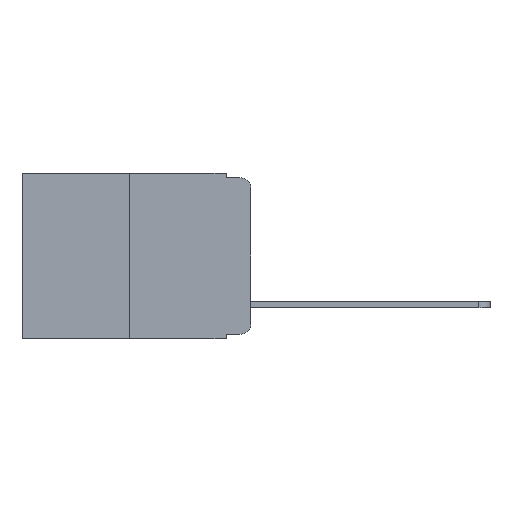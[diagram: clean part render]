
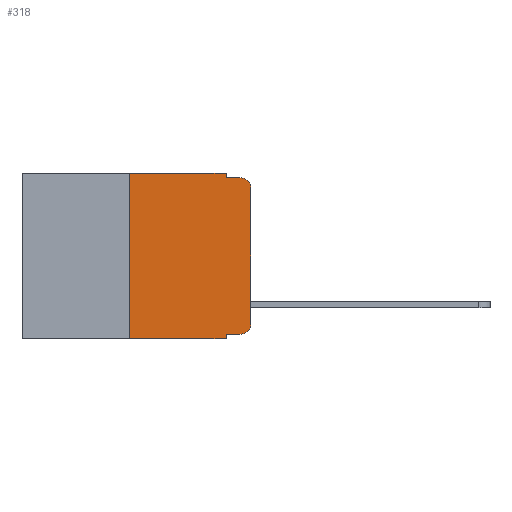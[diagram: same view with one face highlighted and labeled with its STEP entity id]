
A CAD part, left-side view. The second image highlights one B-rep face of the part: STEP entity #318.
In plain terms, the highlighted planar face has unit normal (-1, 0, 0).
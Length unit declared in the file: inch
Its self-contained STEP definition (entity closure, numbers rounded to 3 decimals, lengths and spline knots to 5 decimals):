
#45 = CARTESIAN_POINT ( 'NONE',  ( 0., 0., -0.03 ) ) ;
#90 = DIRECTION ( 'NONE',  ( 0., -1., 0. ) ) ;
#96 = PLANE ( 'NONE',  #7021 ) ;
#160 = ORIENTED_EDGE ( 'NONE', *, *, #5198, .T. ) ;
#318 = ADVANCED_FACE ( 'NONE', ( #749 ), #96, .F. ) ;
#366 = VECTOR ( 'NONE', #1645, 39.37008 ) ;
#488 = VERTEX_POINT ( 'NONE', #9440 ) ;
#749 = FACE_OUTER_BOUND ( 'NONE', #10147, .T. ) ;
#823 = ORIENTED_EDGE ( 'NONE', *, *, #6202, .T. ) ;
#852 = VERTEX_POINT ( 'NONE', #1570 ) ;
#1126 = VERTEX_POINT ( 'NONE', #3689 ) ;
#1153 = LINE ( 'NONE', #7464, #6526 ) ;
#1239 = VERTEX_POINT ( 'NONE', #6737 ) ;
#1570 = CARTESIAN_POINT ( 'NONE',  ( 0., 0.02, -0.01 ) ) ;
#1645 = DIRECTION ( 'NONE',  ( 0., 0., -1. ) ) ;
#1784 = LINE ( 'NONE', #7136, #11660 ) ;
#1896 = CARTESIAN_POINT ( 'NONE',  ( 0., 0., 0. ) ) ;
#2383 = DIRECTION ( 'NONE',  ( 0., 0., 1. ) ) ;
#2514 = CARTESIAN_POINT ( 'NONE',  ( 0., 0.25, 0. ) ) ;
#2850 = VERTEX_POINT ( 'NONE', #11942 ) ;
#3355 = VERTEX_POINT ( 'NONE', #9206 ) ;
#3689 = CARTESIAN_POINT ( 'NONE',  ( 0., 0.051, -0.01 ) ) ;
#3874 = CARTESIAN_POINT ( 'NONE',  ( 0., 0.02, -0.333 ) ) ;
#4204 = VERTEX_POINT ( 'NONE', #45 ) ;
#4306 = DIRECTION ( 'NONE',  ( -1., 0., 0. ) ) ;
#4560 = DIRECTION ( 'NONE',  ( 0., -1., 0. ) ) ;
#4792 = EDGE_CURVE ( 'NONE', #1126, #852, #9647, .T. ) ;
#4904 = CARTESIAN_POINT ( 'NONE',  ( 0., 0.473, -0.343 ) ) ;
#4909 = CARTESIAN_POINT ( 'NONE',  ( 0., 0.051, -0.01 ) ) ;
#5058 = CIRCLE ( 'NONE', #6511, 0.02 ) ;
#5089 = VECTOR ( 'NONE', #8851, 39.37008 ) ;
#5197 = VERTEX_POINT ( 'NONE', #2514 ) ;
#5198 = EDGE_CURVE ( 'NONE', #9395, #4204, #5793, .T. ) ;
#5280 = CIRCLE ( 'NONE', #8051, 0.02 ) ;
#5439 = LINE ( 'NONE', #9256, #12081 ) ;
#5793 = LINE ( 'NONE', #1896, #12102 ) ;
#5828 = VERTEX_POINT ( 'NONE', #3874 ) ;
#6048 = DIRECTION ( 'NONE',  ( 0., -1., 0. ) ) ;
#6202 = EDGE_CURVE ( 'NONE', #4204, #852, #5280, .T. ) ;
#6375 = ORIENTED_EDGE ( 'NONE', *, *, #8945, .T. ) ;
#6511 = AXIS2_PLACEMENT_3D ( 'NONE', #11617, #11629, #6986 ) ;
#6526 = VECTOR ( 'NONE', #8425, 39.37008 ) ;
#6737 = CARTESIAN_POINT ( 'NONE',  ( 0., 0.051, 0. ) ) ;
#6873 = EDGE_CURVE ( 'NONE', #2850, #5197, #5439, .T. ) ;
#6971 = DIRECTION ( 'NONE',  ( 1., 0., 0. ) ) ;
#6986 = DIRECTION ( 'NONE',  ( 0., 0., -1. ) ) ;
#7021 = AXIS2_PLACEMENT_3D ( 'NONE', #7030, #6971, #7131 ) ;
#7030 = CARTESIAN_POINT ( 'NONE',  ( 0., 0.473, 0. ) ) ;
#7092 = ORIENTED_EDGE ( 'NONE', *, *, #8535, .T. ) ;
#7131 = DIRECTION ( 'NONE',  ( 0., 0., -1. ) ) ;
#7136 = CARTESIAN_POINT ( 'NONE',  ( 0., 0.051, -0.333 ) ) ;
#7150 = ORIENTED_EDGE ( 'NONE', *, *, #9022, .F. ) ;
#7186 = ORIENTED_EDGE ( 'NONE', *, *, #11784, .T. ) ;
#7464 = CARTESIAN_POINT ( 'NONE',  ( 0., 0.051, 0. ) ) ;
#8051 = AXIS2_PLACEMENT_3D ( 'NONE', #9296, #4306, #10740 ) ;
#8417 = LINE ( 'NONE', #8868, #366 ) ;
#8425 = DIRECTION ( 'NONE',  ( 0., 0., -1. ) ) ;
#8504 = CARTESIAN_POINT ( 'NONE',  ( 0., 0., -0.313 ) ) ;
#8535 = EDGE_CURVE ( 'NONE', #488, #5828, #1784, .T. ) ;
#8619 = ORIENTED_EDGE ( 'NONE', *, *, #6873, .F. ) ;
#8668 = ORIENTED_EDGE ( 'NONE', *, *, #10211, .F. ) ;
#8851 = DIRECTION ( 'NONE',  ( 0., -1., 0. ) ) ;
#8868 = CARTESIAN_POINT ( 'NONE',  ( 0., 0.051, 0. ) ) ;
#8945 = EDGE_CURVE ( 'NONE', #5828, #9395, #5058, .T. ) ;
#9022 = EDGE_CURVE ( 'NONE', #488, #3355, #8417, .T. ) ;
#9090 = LINE ( 'NONE', #11751, #11078 ) ;
#9206 = CARTESIAN_POINT ( 'NONE',  ( 0., 0.051, -0.343 ) ) ;
#9220 = DIRECTION ( 'NONE',  ( 0., 0., 1. ) ) ;
#9256 = CARTESIAN_POINT ( 'NONE',  ( 0., 0.25, 0. ) ) ;
#9296 = CARTESIAN_POINT ( 'NONE',  ( 0., 0.02, -0.03 ) ) ;
#9395 = VERTEX_POINT ( 'NONE', #8504 ) ;
#9440 = CARTESIAN_POINT ( 'NONE',  ( 0., 0.051, -0.333 ) ) ;
#9647 = LINE ( 'NONE', #4909, #11725 ) ;
#9834 = LINE ( 'NONE', #4904, #5089 ) ;
#10147 = EDGE_LOOP ( 'NONE', ( #160, #823, #11451, #10665, #8668, #8619, #7186, #7150, #7092, #6375 ) ) ;
#10211 = EDGE_CURVE ( 'NONE', #5197, #1239, #9090, .T. ) ;
#10665 = ORIENTED_EDGE ( 'NONE', *, *, #11530, .F. ) ;
#10740 = DIRECTION ( 'NONE',  ( 0., 0., -1. ) ) ;
#11078 = VECTOR ( 'NONE', #90, 39.37008 ) ;
#11451 = ORIENTED_EDGE ( 'NONE', *, *, #4792, .F. ) ;
#11530 = EDGE_CURVE ( 'NONE', #1239, #1126, #1153, .T. ) ;
#11617 = CARTESIAN_POINT ( 'NONE',  ( 0., 0.02, -0.313 ) ) ;
#11629 = DIRECTION ( 'NONE',  ( -1., 0., 0. ) ) ;
#11660 = VECTOR ( 'NONE', #6048, 39.37008 ) ;
#11725 = VECTOR ( 'NONE', #4560, 39.37008 ) ;
#11751 = CARTESIAN_POINT ( 'NONE',  ( 0., 0.473, 0. ) ) ;
#11784 = EDGE_CURVE ( 'NONE', #2850, #3355, #9834, .T. ) ;
#11942 = CARTESIAN_POINT ( 'NONE',  ( 0., 0.25, -0.343 ) ) ;
#12081 = VECTOR ( 'NONE', #9220, 39.37008 ) ;
#12102 = VECTOR ( 'NONE', #2383, 39.37008 ) ;
